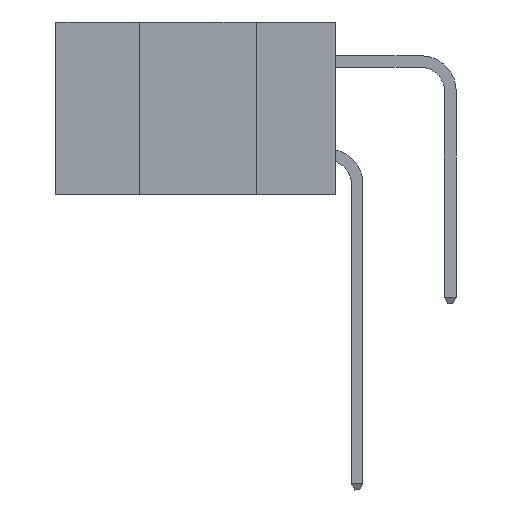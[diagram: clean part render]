
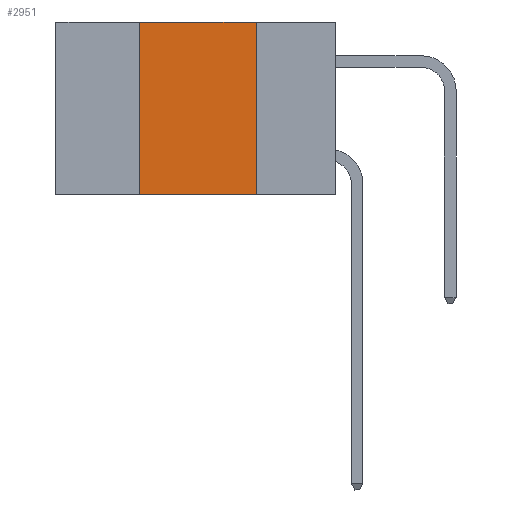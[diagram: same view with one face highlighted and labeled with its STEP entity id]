
A CAD part, left-side view. The second image highlights one B-rep face of the part: STEP entity #2951.
In plain terms, the highlighted planar face has unit normal (-1, 0, 0).
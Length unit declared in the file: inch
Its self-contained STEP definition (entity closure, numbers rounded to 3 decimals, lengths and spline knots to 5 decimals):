
#136 = DIRECTION ( 'NONE',  ( 0., -1., 0. ) ) ;
#812 = LINE ( 'NONE', #9320, #17350 ) ;
#1436 = CARTESIAN_POINT ( 'NONE',  ( 0., 0.17, 0. ) ) ;
#2163 = VERTEX_POINT ( 'NONE', #20386 ) ;
#2762 = LINE ( 'NONE', #9186, #7684 ) ;
#2922 = ORIENTED_EDGE ( 'NONE', *, *, #9625, .F. ) ;
#2951 = ADVANCED_FACE ( 'NONE', ( #12165 ), #20292, .F. ) ;
#3106 = LINE ( 'NONE', #6108, #15430 ) ;
#3444 = EDGE_CURVE ( 'NONE', #2163, #8283, #812, .T. ) ;
#4311 = DIRECTION ( 'NONE',  ( 0., 0., 1. ) ) ;
#4982 = VERTEX_POINT ( 'NONE', #1436 ) ;
#6014 = ORIENTED_EDGE ( 'NONE', *, *, #3444, .T. ) ;
#6108 = CARTESIAN_POINT ( 'NONE',  ( 0., 0.17, 0. ) ) ;
#6341 = CARTESIAN_POINT ( 'NONE',  ( 0., 0.6, 0. ) ) ;
#6653 = ORIENTED_EDGE ( 'NONE', *, *, #14549, .F. ) ;
#7176 = EDGE_CURVE ( 'NONE', #9697, #4982, #11433, .T. ) ;
#7684 = VECTOR ( 'NONE', #4311, 39.37008 ) ;
#8283 = VERTEX_POINT ( 'NONE', #19335 ) ;
#9186 = CARTESIAN_POINT ( 'NONE',  ( 0., 0.42, 0. ) ) ;
#9320 = CARTESIAN_POINT ( 'NONE',  ( 0., 0.6, -0.37 ) ) ;
#9625 = EDGE_CURVE ( 'NONE', #2163, #9697, #2762, .T. ) ;
#9697 = VERTEX_POINT ( 'NONE', #12195 ) ;
#11433 = LINE ( 'NONE', #6341, #15156 ) ;
#12165 = FACE_OUTER_BOUND ( 'NONE', #12247, .T. ) ;
#12186 = AXIS2_PLACEMENT_3D ( 'NONE', #14063, #17251, #18830 ) ;
#12195 = CARTESIAN_POINT ( 'NONE',  ( 0., 0.42, 0. ) ) ;
#12247 = EDGE_LOOP ( 'NONE', ( #6653, #13326, #2922, #6014 ) ) ;
#12902 = DIRECTION ( 'NONE',  ( 0., -1., 0. ) ) ;
#13326 = ORIENTED_EDGE ( 'NONE', *, *, #7176, .F. ) ;
#14063 = CARTESIAN_POINT ( 'NONE',  ( 0., 0.6, 0. ) ) ;
#14549 = EDGE_CURVE ( 'NONE', #4982, #8283, #3106, .T. ) ;
#15156 = VECTOR ( 'NONE', #12902, 39.37008 ) ;
#15430 = VECTOR ( 'NONE', #18561, 39.37008 ) ;
#17251 = DIRECTION ( 'NONE',  ( 1., 0., 0. ) ) ;
#17350 = VECTOR ( 'NONE', #136, 39.37008 ) ;
#18561 = DIRECTION ( 'NONE',  ( 0., 0., -1. ) ) ;
#18830 = DIRECTION ( 'NONE',  ( 0., 0., -1. ) ) ;
#19335 = CARTESIAN_POINT ( 'NONE',  ( 0., 0.17, -0.37 ) ) ;
#20292 = PLANE ( 'NONE',  #12186 ) ;
#20386 = CARTESIAN_POINT ( 'NONE',  ( 0., 0.42, -0.37 ) ) ;
